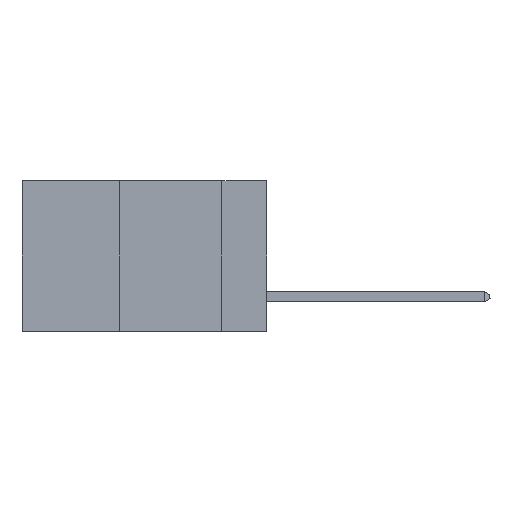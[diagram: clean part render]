
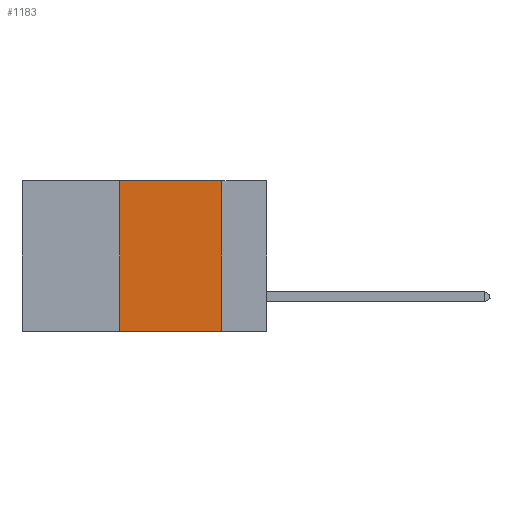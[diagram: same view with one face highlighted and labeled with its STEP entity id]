
A CAD part, left-side view. The second image highlights one B-rep face of the part: STEP entity #1183.
In plain terms, the highlighted planar face has unit normal (-1, 0, 0).
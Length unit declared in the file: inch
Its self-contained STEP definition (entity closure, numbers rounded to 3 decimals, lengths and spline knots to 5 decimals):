
#1183 = ADVANCED_FACE ( 'NONE', ( #17063 ), #24909, .F. ) ;
#1250 = ORIENTED_EDGE ( 'NONE', *, *, #22880, .F. ) ;
#3470 = VECTOR ( 'NONE', #37490, 39.37008 ) ;
#4771 = EDGE_LOOP ( 'NONE', ( #31067, #24299, #1250, #31785 ) ) ;
#9253 = VECTOR ( 'NONE', #23412, 39.37008 ) ;
#10802 = CARTESIAN_POINT ( 'NONE',  ( 0., 0.36, -0.37 ) ) ;
#13243 = CARTESIAN_POINT ( 'NONE',  ( 0., 0.36, 0. ) ) ;
#13485 = DIRECTION ( 'NONE',  ( 0., 0., -1. ) ) ;
#15435 = DIRECTION ( 'NONE',  ( 1., 0., 0. ) ) ;
#16374 = LINE ( 'NONE', #31181, #3470 ) ;
#17063 = FACE_OUTER_BOUND ( 'NONE', #4771, .T. ) ;
#17196 = LINE ( 'NONE', #13243, #31072 ) ;
#19267 = CARTESIAN_POINT ( 'NONE',  ( 0., 0.11, 0. ) ) ;
#20293 = EDGE_CURVE ( 'NONE', #31485, #26965, #16374, .T. ) ;
#21029 = LINE ( 'NONE', #19267, #23418 ) ;
#22055 = DIRECTION ( 'NONE',  ( 0., 0., 1. ) ) ;
#22546 = EDGE_CURVE ( 'NONE', #37823, #26965, #21029, .T. ) ;
#22860 = CARTESIAN_POINT ( 'NONE',  ( 0., 0.6, 0. ) ) ;
#22880 = EDGE_CURVE ( 'NONE', #31485, #34694, #17196, .T. ) ;
#23412 = DIRECTION ( 'NONE',  ( 0., -1., 0. ) ) ;
#23418 = VECTOR ( 'NONE', #13485, 39.37008 ) ;
#24180 = CARTESIAN_POINT ( 'NONE',  ( 0., 0.11, -0.37 ) ) ;
#24299 = ORIENTED_EDGE ( 'NONE', *, *, #38092, .F. ) ;
#24909 = PLANE ( 'NONE',  #34272 ) ;
#26965 = VERTEX_POINT ( 'NONE', #24180 ) ;
#27735 = CARTESIAN_POINT ( 'NONE',  ( 0., 0.6, 0. ) ) ;
#27813 = CARTESIAN_POINT ( 'NONE',  ( 0., 0.36, 0. ) ) ;
#29864 = LINE ( 'NONE', #22860, #9253 ) ;
#30818 = CARTESIAN_POINT ( 'NONE',  ( 0., 0.11, 0. ) ) ;
#30842 = DIRECTION ( 'NONE',  ( 0., 0., -1. ) ) ;
#31067 = ORIENTED_EDGE ( 'NONE', *, *, #22546, .F. ) ;
#31072 = VECTOR ( 'NONE', #22055, 39.37008 ) ;
#31181 = CARTESIAN_POINT ( 'NONE',  ( 0., 0.6, -0.37 ) ) ;
#31485 = VERTEX_POINT ( 'NONE', #10802 ) ;
#31785 = ORIENTED_EDGE ( 'NONE', *, *, #20293, .T. ) ;
#34272 = AXIS2_PLACEMENT_3D ( 'NONE', #27735, #15435, #30842 ) ;
#34694 = VERTEX_POINT ( 'NONE', #27813 ) ;
#37490 = DIRECTION ( 'NONE',  ( 0., -1., 0. ) ) ;
#37823 = VERTEX_POINT ( 'NONE', #30818 ) ;
#38092 = EDGE_CURVE ( 'NONE', #34694, #37823, #29864, .T. ) ;
